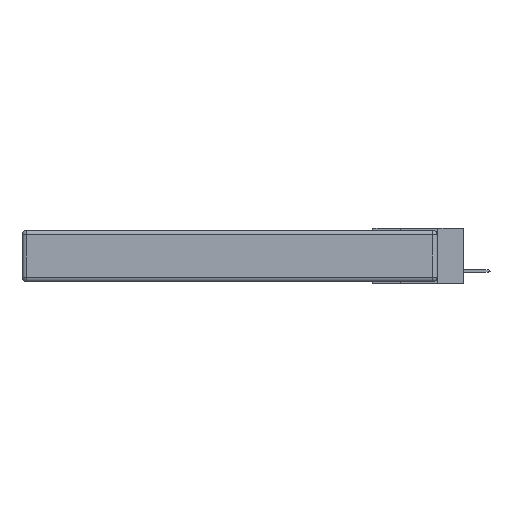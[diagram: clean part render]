
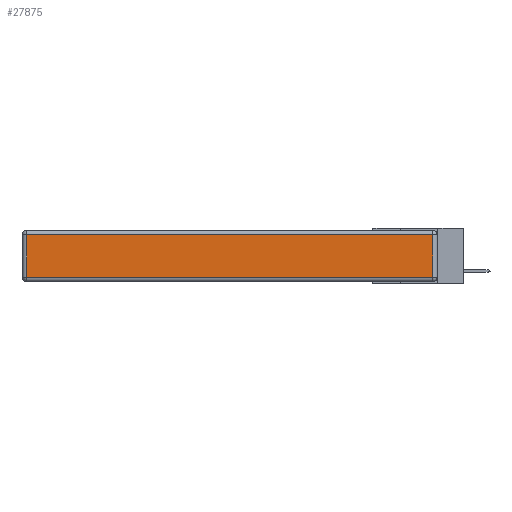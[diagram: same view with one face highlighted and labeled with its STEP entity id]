
A CAD part, left-side view. The second image highlights one B-rep face of the part: STEP entity #27875.
In plain terms, the highlighted planar face has unit normal (-1, 0, 0).
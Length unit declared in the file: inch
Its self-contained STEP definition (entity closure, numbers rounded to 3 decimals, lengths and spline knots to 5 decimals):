
#999 = PLANE ( 'NONE',  #14659 ) ;
#1184 = CARTESIAN_POINT ( 'NONE',  ( 0., 0., -0.343 ) ) ;
#4300 = VERTEX_POINT ( 'NONE', #28174 ) ;
#4789 = FACE_OUTER_BOUND ( 'NONE', #19272, .T. ) ;
#5611 = DIRECTION ( 'NONE',  ( 0., -1., 0. ) ) ;
#6125 = CARTESIAN_POINT ( 'NONE',  ( 0., 0.03, -0.313 ) ) ;
#7267 = CARTESIAN_POINT ( 'NONE',  ( 0., 0.03, -0.03 ) ) ;
#7588 = EDGE_CURVE ( 'NONE', #9262, #4300, #11561, .T. ) ;
#8682 = CARTESIAN_POINT ( 'NONE',  ( 0., 2.72, -0.03 ) ) ;
#9212 = LINE ( 'NONE', #21013, #12006 ) ;
#9262 = VERTEX_POINT ( 'NONE', #8682 ) ;
#9273 = ORIENTED_EDGE ( 'NONE', *, *, #26649, .T. ) ;
#10232 = VERTEX_POINT ( 'NONE', #6125 ) ;
#11561 = LINE ( 'NONE', #12932, #24388 ) ;
#11974 = EDGE_CURVE ( 'NONE', #4300, #10232, #9212, .T. ) ;
#12006 = VECTOR ( 'NONE', #5611, 39.37008 ) ;
#12932 = CARTESIAN_POINT ( 'NONE',  ( 0., 2.72, -0.343 ) ) ;
#14531 = DIRECTION ( 'NONE',  ( 0., 0., 1. ) ) ;
#14659 = AXIS2_PLACEMENT_3D ( 'NONE', #1184, #18621, #16680 ) ;
#16383 = VECTOR ( 'NONE', #28328, 39.37008 ) ;
#16680 = DIRECTION ( 'NONE',  ( 0., 0., 1. ) ) ;
#17750 = ORIENTED_EDGE ( 'NONE', *, *, #7588, .T. ) ;
#18621 = DIRECTION ( 'NONE',  ( -1., 0., 0. ) ) ;
#18881 = CARTESIAN_POINT ( 'NONE',  ( 0., 0.03, -0.343 ) ) ;
#19272 = EDGE_LOOP ( 'NONE', ( #22803, #9273, #25356, #17750 ) ) ;
#19359 = CARTESIAN_POINT ( 'NONE',  ( 0., 2.75, -0.03 ) ) ;
#19410 = EDGE_CURVE ( 'NONE', #28070, #9262, #25720, .T. ) ;
#21013 = CARTESIAN_POINT ( 'NONE',  ( 0., 0., -0.313 ) ) ;
#22803 = ORIENTED_EDGE ( 'NONE', *, *, #11974, .T. ) ;
#24388 = VECTOR ( 'NONE', #26299, 39.37008 ) ;
#24630 = LINE ( 'NONE', #18881, #26344 ) ;
#25356 = ORIENTED_EDGE ( 'NONE', *, *, #19410, .T. ) ;
#25720 = LINE ( 'NONE', #19359, #16383 ) ;
#26299 = DIRECTION ( 'NONE',  ( 0., 0., -1. ) ) ;
#26344 = VECTOR ( 'NONE', #14531, 39.37008 ) ;
#26649 = EDGE_CURVE ( 'NONE', #10232, #28070, #24630, .T. ) ;
#27875 = ADVANCED_FACE ( 'NONE', ( #4789 ), #999, .T. ) ;
#28070 = VERTEX_POINT ( 'NONE', #7267 ) ;
#28174 = CARTESIAN_POINT ( 'NONE',  ( 0., 2.72, -0.313 ) ) ;
#28328 = DIRECTION ( 'NONE',  ( 0., 1., 0. ) ) ;
